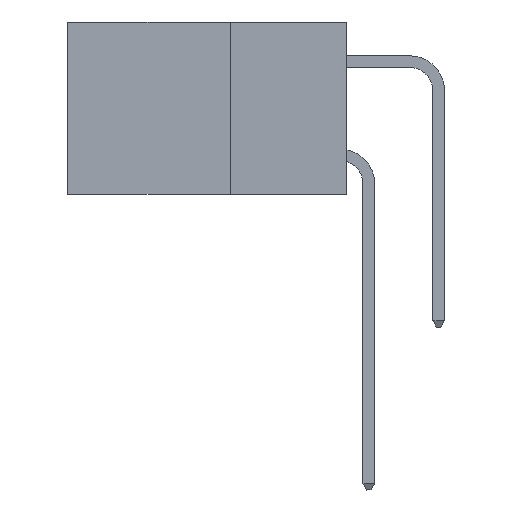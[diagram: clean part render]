
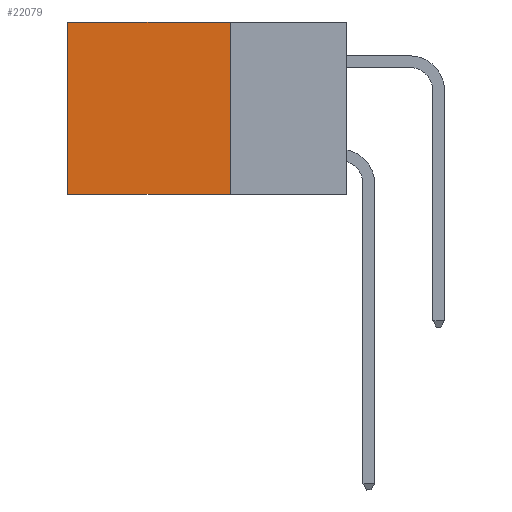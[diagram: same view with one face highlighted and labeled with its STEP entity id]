
A CAD part, left-side view. The second image highlights one B-rep face of the part: STEP entity #22079.
In plain terms, the highlighted planar face has unit normal (-1, 0, 0).
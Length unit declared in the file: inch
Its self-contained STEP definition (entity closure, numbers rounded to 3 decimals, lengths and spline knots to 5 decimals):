
#735 = ORIENTED_EDGE ( 'NONE', *, *, #7085, .T. ) ;
#2227 = EDGE_CURVE ( 'NONE', #16261, #19260, #14515, .T. ) ;
#5044 = ORIENTED_EDGE ( 'NONE', *, *, #2227, .F. ) ;
#6771 = CARTESIAN_POINT ( 'NONE',  ( 0.2875, 0.25, -0.37 ) ) ;
#7085 = EDGE_CURVE ( 'NONE', #28124, #14136, #11470, .T. ) ;
#7199 = EDGE_LOOP ( 'NONE', ( #7320, #5044, #32273, #735 ) ) ;
#7320 = ORIENTED_EDGE ( 'NONE', *, *, #21964, .T. ) ;
#9185 = PLANE ( 'NONE',  #23729 ) ;
#10981 = CARTESIAN_POINT ( 'NONE',  ( 0.2875, 0.6, 0. ) ) ;
#11151 = CARTESIAN_POINT ( 'NONE',  ( 0.2875, 0.25, 0. ) ) ;
#11470 = LINE ( 'NONE', #18880, #16692 ) ;
#11811 = FACE_OUTER_BOUND ( 'NONE', #7199, .T. ) ;
#12564 = VECTOR ( 'NONE', #25946, 39.37008 ) ;
#12984 = DIRECTION ( 'NONE',  ( 0., 0., -1. ) ) ;
#14136 = VERTEX_POINT ( 'NONE', #27839 ) ;
#14515 = LINE ( 'NONE', #6771, #26429 ) ;
#15963 = CARTESIAN_POINT ( 'NONE',  ( 0.2875, 0.25, 0. ) ) ;
#16261 = VERTEX_POINT ( 'NONE', #29259 ) ;
#16692 = VECTOR ( 'NONE', #28866, 39.37008 ) ;
#16697 = EDGE_CURVE ( 'NONE', #28124, #16261, #28400, .T. ) ;
#16826 = DIRECTION ( 'NONE',  ( 0., 1., 0. ) ) ;
#17436 = VECTOR ( 'NONE', #12984, 39.37008 ) ;
#18880 = CARTESIAN_POINT ( 'NONE',  ( 0.2875, 0.25, 0. ) ) ;
#18885 = DIRECTION ( 'NONE',  ( 0., 0., -1. ) ) ;
#19221 = DIRECTION ( 'NONE',  ( 1., 0., 0. ) ) ;
#19260 = VERTEX_POINT ( 'NONE', #25565 ) ;
#21964 = EDGE_CURVE ( 'NONE', #14136, #19260, #25618, .T. ) ;
#22079 = ADVANCED_FACE ( 'NONE', ( #11811 ), #9185, .F. ) ;
#23729 = AXIS2_PLACEMENT_3D ( 'NONE', #23971, #19221, #18885 ) ;
#23971 = CARTESIAN_POINT ( 'NONE',  ( 0.2875, 0.25, 0. ) ) ;
#25565 = CARTESIAN_POINT ( 'NONE',  ( 0.2875, 0.6, -0.37 ) ) ;
#25618 = LINE ( 'NONE', #10981, #17436 ) ;
#25946 = DIRECTION ( 'NONE',  ( 0., 0., -1. ) ) ;
#26429 = VECTOR ( 'NONE', #16826, 39.37008 ) ;
#27839 = CARTESIAN_POINT ( 'NONE',  ( 0.2875, 0.6, 0. ) ) ;
#28124 = VERTEX_POINT ( 'NONE', #11151 ) ;
#28400 = LINE ( 'NONE', #15963, #12564 ) ;
#28866 = DIRECTION ( 'NONE',  ( 0., 1., 0. ) ) ;
#29259 = CARTESIAN_POINT ( 'NONE',  ( 0.2875, 0.25, -0.37 ) ) ;
#32273 = ORIENTED_EDGE ( 'NONE', *, *, #16697, .F. ) ;
